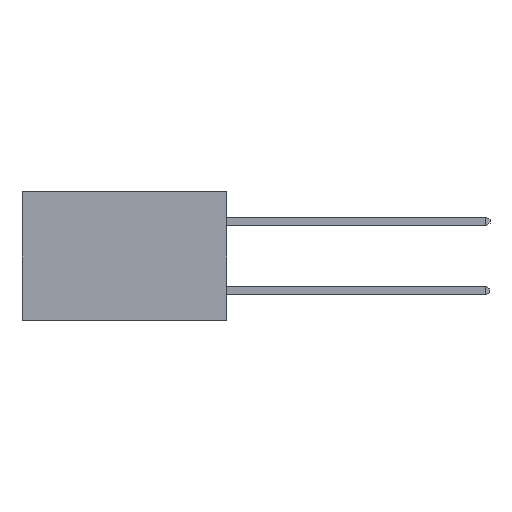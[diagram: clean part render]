
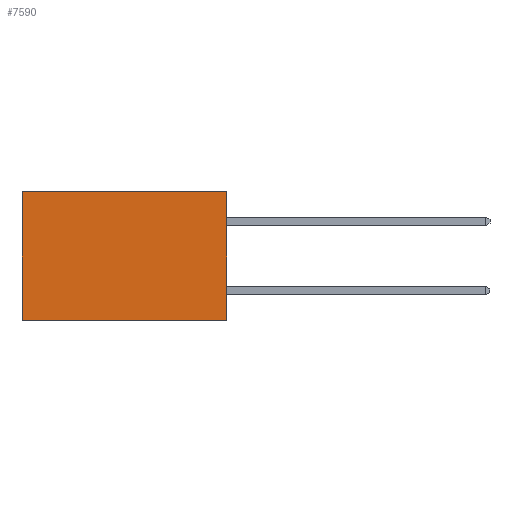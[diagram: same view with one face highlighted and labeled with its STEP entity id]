
A CAD part, left-side view. The second image highlights one B-rep face of the part: STEP entity #7590.
In plain terms, the highlighted planar face has unit normal (-1, 0, 0).
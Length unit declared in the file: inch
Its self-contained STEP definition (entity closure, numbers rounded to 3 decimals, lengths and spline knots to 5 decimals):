
#653 = CARTESIAN_POINT ( 'NONE',  ( 0.277, 0.59, -0.37 ) ) ;
#1437 = CARTESIAN_POINT ( 'NONE',  ( 0.277, 0.59, -0.37 ) ) ;
#1470 = DIRECTION ( 'NONE',  ( 0., 1., 0. ) ) ;
#2620 = CARTESIAN_POINT ( 'NONE',  ( 0.277, 0., -0.37 ) ) ;
#2795 = AXIS2_PLACEMENT_3D ( 'NONE', #11422, #14920, #7820 ) ;
#2870 = VERTEX_POINT ( 'NONE', #1437 ) ;
#3310 = VERTEX_POINT ( 'NONE', #5422 ) ;
#5170 = ORIENTED_EDGE ( 'NONE', *, *, #9560, .T. ) ;
#5324 = VECTOR ( 'NONE', #5877, 39.37008 ) ;
#5422 = CARTESIAN_POINT ( 'NONE',  ( 0.277, 0., 0. ) ) ;
#5478 = VERTEX_POINT ( 'NONE', #11741 ) ;
#5877 = DIRECTION ( 'NONE',  ( 0., 0., -1. ) ) ;
#6105 = VECTOR ( 'NONE', #6347, 39.37008 ) ;
#6321 = ORIENTED_EDGE ( 'NONE', *, *, #15128, .T. ) ;
#6347 = DIRECTION ( 'NONE',  ( 0., 0., -1. ) ) ;
#7458 = VECTOR ( 'NONE', #13954, 39.37008 ) ;
#7590 = ADVANCED_FACE ( 'NONE', ( #14258 ), #14882, .F. ) ;
#7820 = DIRECTION ( 'NONE',  ( 0., 0., -1. ) ) ;
#7989 = CARTESIAN_POINT ( 'NONE',  ( 0.277, 0., 0. ) ) ;
#8853 = ORIENTED_EDGE ( 'NONE', *, *, #14951, .F. ) ;
#9381 = LINE ( 'NONE', #11241, #6105 ) ;
#9560 = EDGE_CURVE ( 'NONE', #5478, #2870, #14899, .T. ) ;
#9896 = EDGE_LOOP ( 'NONE', ( #5170, #14759, #8853, #6321 ) ) ;
#10923 = VECTOR ( 'NONE', #1470, 39.37008 ) ;
#11241 = CARTESIAN_POINT ( 'NONE',  ( 0.277, 0., -0.37 ) ) ;
#11290 = LINE ( 'NONE', #11486, #10923 ) ;
#11422 = CARTESIAN_POINT ( 'NONE',  ( 0.277, 0., -0.37 ) ) ;
#11486 = CARTESIAN_POINT ( 'NONE',  ( 0.277, 0., -0.37 ) ) ;
#11741 = CARTESIAN_POINT ( 'NONE',  ( 0.277, 0.59, 0. ) ) ;
#11977 = VERTEX_POINT ( 'NONE', #2620 ) ;
#13954 = DIRECTION ( 'NONE',  ( 0., 1., 0. ) ) ;
#14206 = LINE ( 'NONE', #7989, #7458 ) ;
#14224 = EDGE_CURVE ( 'NONE', #11977, #2870, #11290, .T. ) ;
#14258 = FACE_OUTER_BOUND ( 'NONE', #9896, .T. ) ;
#14759 = ORIENTED_EDGE ( 'NONE', *, *, #14224, .F. ) ;
#14882 = PLANE ( 'NONE',  #2795 ) ;
#14899 = LINE ( 'NONE', #653, #5324 ) ;
#14920 = DIRECTION ( 'NONE',  ( 1., 0., 0. ) ) ;
#14951 = EDGE_CURVE ( 'NONE', #3310, #11977, #9381, .T. ) ;
#15128 = EDGE_CURVE ( 'NONE', #3310, #5478, #14206, .T. ) ;
